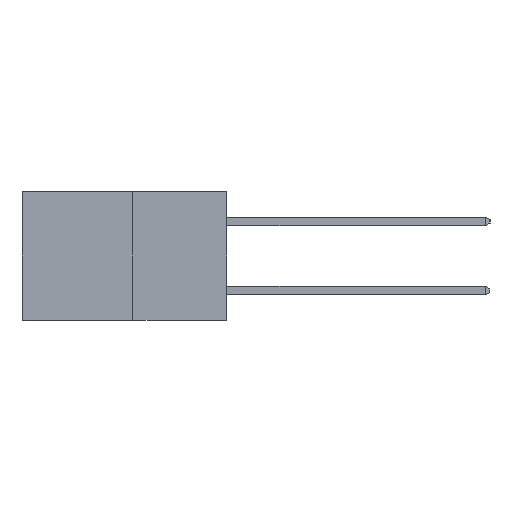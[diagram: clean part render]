
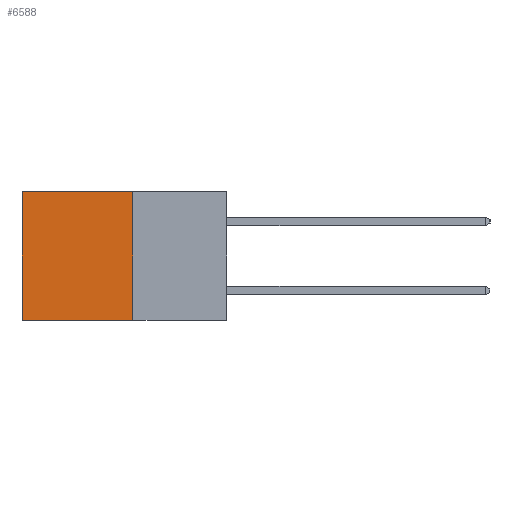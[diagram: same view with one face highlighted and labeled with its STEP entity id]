
A CAD part, left-side view. The second image highlights one B-rep face of the part: STEP entity #6588.
In plain terms, the highlighted planar face has unit normal (-1, 0, 0).
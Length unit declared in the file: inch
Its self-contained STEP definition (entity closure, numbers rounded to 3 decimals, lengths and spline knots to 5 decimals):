
#127 = VECTOR ( 'NONE', #5515, 39.37008 ) ;
#2011 = CARTESIAN_POINT ( 'NONE',  ( 0.277, 0.27, -0.37 ) ) ;
#2055 = VERTEX_POINT ( 'NONE', #9069 ) ;
#3035 = ORIENTED_EDGE ( 'NONE', *, *, #3226, .T. ) ;
#3208 = ORIENTED_EDGE ( 'NONE', *, *, #16262, .F. ) ;
#3226 = EDGE_CURVE ( 'NONE', #2055, #19170, #6466, .T. ) ;
#4345 = ORIENTED_EDGE ( 'NONE', *, *, #13816, .F. ) ;
#4756 = CARTESIAN_POINT ( 'NONE',  ( 0.277, 0.59, -0.37 ) ) ;
#5006 = ORIENTED_EDGE ( 'NONE', *, *, #6625, .T. ) ;
#5071 = DIRECTION ( 'NONE',  ( 0., 1., 0. ) ) ;
#5515 = DIRECTION ( 'NONE',  ( 0., 0., -1. ) ) ;
#6466 = LINE ( 'NONE', #16219, #13719 ) ;
#6588 = ADVANCED_FACE ( 'NONE', ( #19342 ), #7875, .F. ) ;
#6625 = EDGE_CURVE ( 'NONE', #7874, #2055, #16409, .T. ) ;
#7484 = CARTESIAN_POINT ( 'NONE',  ( 0.277, 0.27, 0. ) ) ;
#7510 = CARTESIAN_POINT ( 'NONE',  ( 0.277, 0.27, 0. ) ) ;
#7599 = DIRECTION ( 'NONE',  ( 0., 1., 0. ) ) ;
#7813 = DIRECTION ( 'NONE',  ( 0., 0., -1. ) ) ;
#7850 = DIRECTION ( 'NONE',  ( 1., 0., 0. ) ) ;
#7860 = CARTESIAN_POINT ( 'NONE',  ( 0.277, 0.27, -0.37 ) ) ;
#7874 = VERTEX_POINT ( 'NONE', #7484 ) ;
#7875 = PLANE ( 'NONE',  #8082 ) ;
#8082 = AXIS2_PLACEMENT_3D ( 'NONE', #7860, #7850, #7813 ) ;
#8411 = LINE ( 'NONE', #19137, #127 ) ;
#8798 = CARTESIAN_POINT ( 'NONE',  ( 0.277, 0.27, -0.37 ) ) ;
#9069 = CARTESIAN_POINT ( 'NONE',  ( 0.277, 0.59, 0. ) ) ;
#10928 = VECTOR ( 'NONE', #7599, 39.37008 ) ;
#11303 = EDGE_LOOP ( 'NONE', ( #3035, #3208, #4345, #5006 ) ) ;
#12945 = VERTEX_POINT ( 'NONE', #8798 ) ;
#13719 = VECTOR ( 'NONE', #16007, 39.37008 ) ;
#13816 = EDGE_CURVE ( 'NONE', #7874, #12945, #8411, .T. ) ;
#14410 = VECTOR ( 'NONE', #5071, 39.37008 ) ;
#16007 = DIRECTION ( 'NONE',  ( 0., 0., -1. ) ) ;
#16219 = CARTESIAN_POINT ( 'NONE',  ( 0.277, 0.59, -0.37 ) ) ;
#16262 = EDGE_CURVE ( 'NONE', #12945, #19170, #19420, .T. ) ;
#16409 = LINE ( 'NONE', #7510, #10928 ) ;
#19137 = CARTESIAN_POINT ( 'NONE',  ( 0.277, 0.27, -0.37 ) ) ;
#19170 = VERTEX_POINT ( 'NONE', #4756 ) ;
#19342 = FACE_OUTER_BOUND ( 'NONE', #11303, .T. ) ;
#19420 = LINE ( 'NONE', #2011, #14410 ) ;
